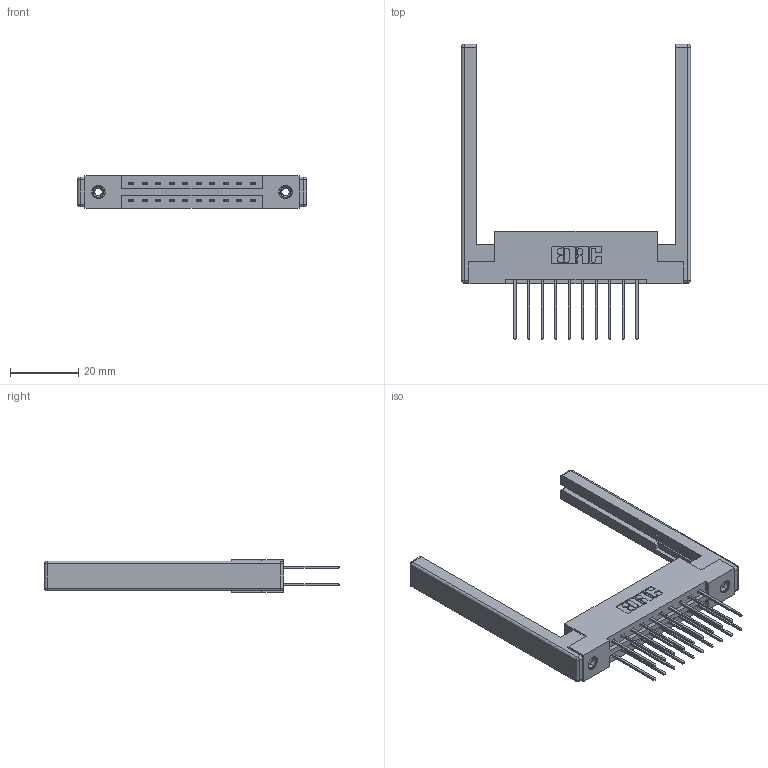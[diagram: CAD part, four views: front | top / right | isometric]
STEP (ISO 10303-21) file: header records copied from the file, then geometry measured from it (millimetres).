
FILE_DESCRIPTION (( 'STEP AP203' ), '1' );
FILE_NAME ('387-020-542-268.STEP', '2019-10-16T15:35:21', ( '' ), ( '' ), 'SwSTEP 2.0', 'SolidWorks 2016', '' );
FILE_SCHEMA (( 'CONFIG_CONTROL_DESIGN' ));
Length unit declared in the file: inch
Products named in the file (5): 345-250-001_345-250-001-102; 387-020-542-268; 337 Part_Flush Mounting Lugs - 0.156 Dia-TI; 307-220-068; 345-292-001_345-293-142
Assembly tree (25 placements, depth 2):
  387-020-542-268
    337 Part_Flush Mounting Lugs - 0.156 Dia-TI
    345-292-001_345-293-142  x20
    345-250-001_345-250-001-102  x2
    307-220-068  x2
Bounding box: 67.06 x 86.37 x 9.4 mm (x, y, z)
Volume: 11119 mm3; surface area: 11801.3 mm2
Topology: 25 solids, 25 shells, 1348 faces, 3921 edges, 2566 vertices
Faces by surface type: plane 918, cylinder 406, cone 12, sphere 8, torus 4
Entity records: 14670 total; most frequent: CARTESIAN_POINT 2463, ORIENTED_EDGE 2388, DIRECTION 2224, EDGE_CURVE 1194, LINE 1016, VECTOR 1016, VERTEX_POINT 786, AXIS2_PLACEMENT_3D 604
